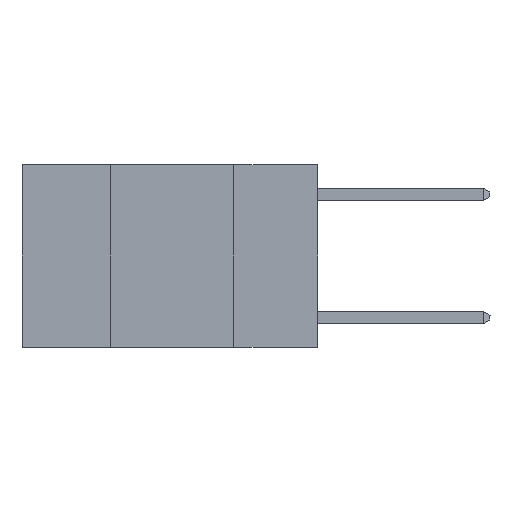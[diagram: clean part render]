
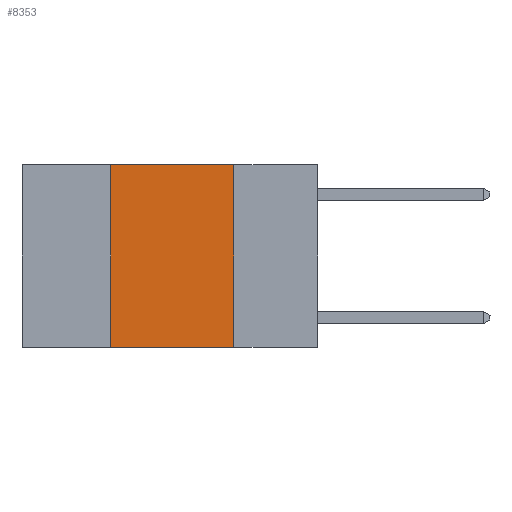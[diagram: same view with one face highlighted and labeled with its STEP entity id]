
A CAD part, left-side view. The second image highlights one B-rep face of the part: STEP entity #8353.
In plain terms, the highlighted planar face has unit normal (-1, 0, 0).
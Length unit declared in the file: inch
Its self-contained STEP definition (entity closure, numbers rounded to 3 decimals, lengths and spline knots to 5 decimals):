
#411 = DIRECTION ( 'NONE',  ( 0., 0., 1. ) ) ;
#475 = CARTESIAN_POINT ( 'NONE',  ( 0., 0.17, 0. ) ) ;
#566 = ORIENTED_EDGE ( 'NONE', *, *, #9065, .F. ) ;
#599 = ORIENTED_EDGE ( 'NONE', *, *, #6265, .F. ) ;
#605 = CARTESIAN_POINT ( 'NONE',  ( 0., 0.42, -0.37 ) ) ;
#621 = ORIENTED_EDGE ( 'NONE', *, *, #1866, .F. ) ;
#630 = ORIENTED_EDGE ( 'NONE', *, *, #4735, .T. ) ;
#649 = VERTEX_POINT ( 'NONE', #5038 ) ;
#875 = VERTEX_POINT ( 'NONE', #7460 ) ;
#1864 = VECTOR ( 'NONE', #6197, 39.37008 ) ;
#1866 = EDGE_CURVE ( 'NONE', #4778, #875, #7001, .T. ) ;
#2071 = CARTESIAN_POINT ( 'NONE',  ( 0., 0.17, -0.37 ) ) ;
#2261 = FACE_OUTER_BOUND ( 'NONE', #6984, .T. ) ;
#3211 = DIRECTION ( 'NONE',  ( 0., -1., 0. ) ) ;
#3994 = LINE ( 'NONE', #5712, #10507 ) ;
#4597 = DIRECTION ( 'NONE',  ( 1., 0., 0. ) ) ;
#4735 = EDGE_CURVE ( 'NONE', #4778, #8358, #3994, .T. ) ;
#4778 = VERTEX_POINT ( 'NONE', #605 ) ;
#5038 = CARTESIAN_POINT ( 'NONE',  ( 0., 0.17, 0. ) ) ;
#5364 = CARTESIAN_POINT ( 'NONE',  ( 0., 0.42, 0. ) ) ;
#5638 = LINE ( 'NONE', #7509, #7287 ) ;
#5712 = CARTESIAN_POINT ( 'NONE',  ( 0., 0.6, -0.37 ) ) ;
#6134 = PLANE ( 'NONE',  #8129 ) ;
#6197 = DIRECTION ( 'NONE',  ( 0., 0., -1. ) ) ;
#6265 = EDGE_CURVE ( 'NONE', #875, #649, #5638, .T. ) ;
#6984 = EDGE_LOOP ( 'NONE', ( #566, #599, #621, #630 ) ) ;
#7001 = LINE ( 'NONE', #5364, #9189 ) ;
#7287 = VECTOR ( 'NONE', #8338, 39.37008 ) ;
#7460 = CARTESIAN_POINT ( 'NONE',  ( 0., 0.42, 0. ) ) ;
#7509 = CARTESIAN_POINT ( 'NONE',  ( 0., 0.6, 0. ) ) ;
#8129 = AXIS2_PLACEMENT_3D ( 'NONE', #9497, #4597, #10304 ) ;
#8338 = DIRECTION ( 'NONE',  ( 0., -1., 0. ) ) ;
#8353 = ADVANCED_FACE ( 'NONE', ( #2261 ), #6134, .F. ) ;
#8358 = VERTEX_POINT ( 'NONE', #2071 ) ;
#9065 = EDGE_CURVE ( 'NONE', #649, #8358, #10282, .T. ) ;
#9189 = VECTOR ( 'NONE', #411, 39.37008 ) ;
#9497 = CARTESIAN_POINT ( 'NONE',  ( 0., 0.6, 0. ) ) ;
#10282 = LINE ( 'NONE', #475, #1864 ) ;
#10304 = DIRECTION ( 'NONE',  ( 0., 0., -1. ) ) ;
#10507 = VECTOR ( 'NONE', #3211, 39.37008 ) ;
